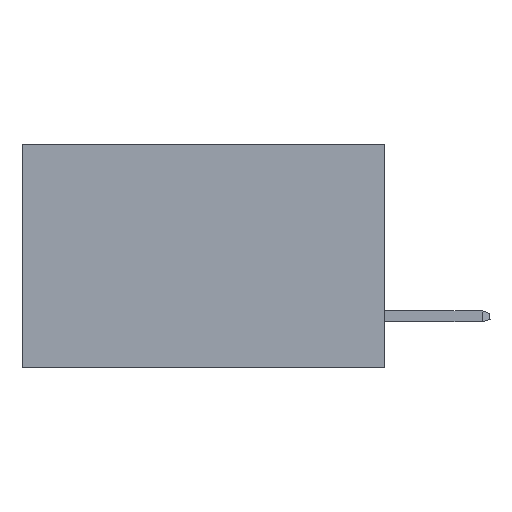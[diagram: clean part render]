
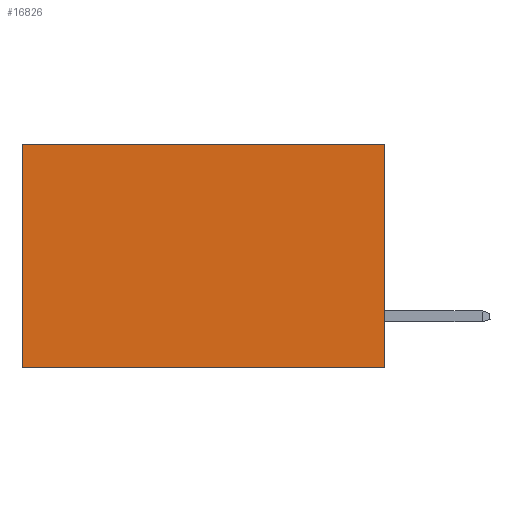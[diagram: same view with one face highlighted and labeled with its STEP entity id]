
A CAD part, left-side view. The second image highlights one B-rep face of the part: STEP entity #16826.
In plain terms, the highlighted planar face has unit normal (-1, 0, 0).
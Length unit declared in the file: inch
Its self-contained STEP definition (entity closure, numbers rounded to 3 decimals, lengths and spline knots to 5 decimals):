
#1711 = DIRECTION ( 'NONE',  ( 0., 0., -1. ) ) ;
#4152 = LINE ( 'NONE', #12330, #15574 ) ;
#4745 = FACE_OUTER_BOUND ( 'NONE', #12275, .T. ) ;
#4919 = VECTOR ( 'NONE', #25164, 39.37008 ) ;
#7668 = DIRECTION ( 'NONE',  ( 0., 1., 0. ) ) ;
#8080 = VERTEX_POINT ( 'NONE', #21603 ) ;
#8622 = CARTESIAN_POINT ( 'NONE',  ( 0.298, 0.6, -0.37 ) ) ;
#8942 = PLANE ( 'NONE',  #14903 ) ;
#9171 = VECTOR ( 'NONE', #26249, 39.37008 ) ;
#9204 = ORIENTED_EDGE ( 'NONE', *, *, #26164, .F. ) ;
#9825 = EDGE_CURVE ( 'NONE', #10934, #8080, #23140, .T. ) ;
#10505 = LINE ( 'NONE', #17606, #9171 ) ;
#10934 = VERTEX_POINT ( 'NONE', #21125 ) ;
#11464 = CARTESIAN_POINT ( 'NONE',  ( 0.298, 0., 0. ) ) ;
#12275 = EDGE_LOOP ( 'NONE', ( #18952, #9204, #21746, #20423 ) ) ;
#12330 = CARTESIAN_POINT ( 'NONE',  ( 0.298, 0., 0. ) ) ;
#14903 = AXIS2_PLACEMENT_3D ( 'NONE', #11464, #24026, #15404 ) ;
#15387 = VECTOR ( 'NONE', #7668, 39.37008 ) ;
#15404 = DIRECTION ( 'NONE',  ( 0., 0., -1. ) ) ;
#15574 = VECTOR ( 'NONE', #1711, 39.37008 ) ;
#16826 = ADVANCED_FACE ( 'NONE', ( #4745 ), #8942, .F. ) ;
#17606 = CARTESIAN_POINT ( 'NONE',  ( 0.298, 0.6, 0. ) ) ;
#17970 = VERTEX_POINT ( 'NONE', #8622 ) ;
#18094 = LINE ( 'NONE', #22644, #15387 ) ;
#18952 = ORIENTED_EDGE ( 'NONE', *, *, #23204, .T. ) ;
#20423 = ORIENTED_EDGE ( 'NONE', *, *, #9825, .T. ) ;
#20690 = VERTEX_POINT ( 'NONE', #27666 ) ;
#21125 = CARTESIAN_POINT ( 'NONE',  ( 0.298, 0., 0. ) ) ;
#21603 = CARTESIAN_POINT ( 'NONE',  ( 0.298, 0.6, 0. ) ) ;
#21746 = ORIENTED_EDGE ( 'NONE', *, *, #21769, .F. ) ;
#21769 = EDGE_CURVE ( 'NONE', #10934, #20690, #4152, .T. ) ;
#22644 = CARTESIAN_POINT ( 'NONE',  ( 0.298, 0., -0.37 ) ) ;
#23140 = LINE ( 'NONE', #24784, #4919 ) ;
#23204 = EDGE_CURVE ( 'NONE', #8080, #17970, #10505, .T. ) ;
#24026 = DIRECTION ( 'NONE',  ( 1., 0., 0. ) ) ;
#24784 = CARTESIAN_POINT ( 'NONE',  ( 0.298, 0., 0. ) ) ;
#25164 = DIRECTION ( 'NONE',  ( 0., 1., 0. ) ) ;
#26164 = EDGE_CURVE ( 'NONE', #20690, #17970, #18094, .T. ) ;
#26249 = DIRECTION ( 'NONE',  ( 0., 0., -1. ) ) ;
#27666 = CARTESIAN_POINT ( 'NONE',  ( 0.298, 0., -0.37 ) ) ;
